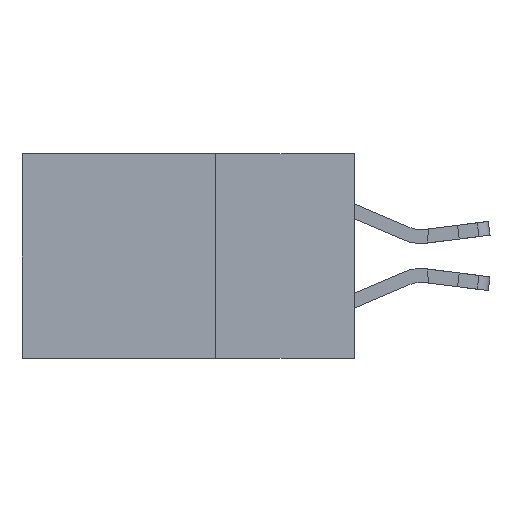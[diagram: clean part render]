
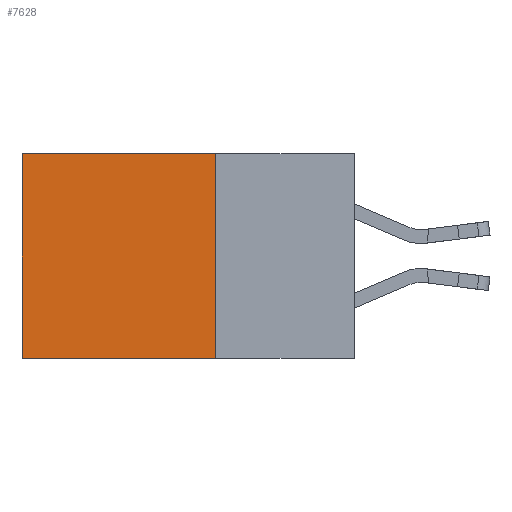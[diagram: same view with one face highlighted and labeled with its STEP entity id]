
A CAD part, left-side view. The second image highlights one B-rep face of the part: STEP entity #7628.
In plain terms, the highlighted planar face has unit normal (-1, 0, 0).
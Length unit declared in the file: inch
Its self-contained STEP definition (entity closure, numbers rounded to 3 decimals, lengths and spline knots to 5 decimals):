
#179 = ORIENTED_EDGE ( 'NONE', *, *, #23772, .T. ) ;
#721 = VECTOR ( 'NONE', #7195, 39.37008 ) ;
#1324 = LINE ( 'NONE', #23699, #721 ) ;
#1481 = DIRECTION ( 'NONE',  ( 0., 0., -1. ) ) ;
#2876 = VERTEX_POINT ( 'NONE', #16165 ) ;
#3820 = CARTESIAN_POINT ( 'NONE',  ( 0.2615, 0.25, -0.37 ) ) ;
#3831 = LINE ( 'NONE', #6799, #17981 ) ;
#3905 = DIRECTION ( 'NONE',  ( 0., 1., 0. ) ) ;
#5344 = EDGE_CURVE ( 'NONE', #5676, #2876, #20279, .T. ) ;
#5606 = VECTOR ( 'NONE', #3905, 39.37008 ) ;
#5676 = VERTEX_POINT ( 'NONE', #17682 ) ;
#6683 = CARTESIAN_POINT ( 'NONE',  ( 0.2615, 0.25, 0. ) ) ;
#6799 = CARTESIAN_POINT ( 'NONE',  ( 0.2615, 0.6, -0.37 ) ) ;
#7195 = DIRECTION ( 'NONE',  ( 0., 0., -1. ) ) ;
#7628 = ADVANCED_FACE ( 'NONE', ( #11336 ), #19925, .F. ) ;
#8099 = EDGE_LOOP ( 'NONE', ( #19903, #8812, #15203, #179 ) ) ;
#8812 = ORIENTED_EDGE ( 'NONE', *, *, #5344, .F. ) ;
#9086 = VERTEX_POINT ( 'NONE', #14521 ) ;
#11336 = FACE_OUTER_BOUND ( 'NONE', #8099, .T. ) ;
#12271 = VECTOR ( 'NONE', #17684, 39.37008 ) ;
#12656 = DIRECTION ( 'NONE',  ( 1., 0., 0. ) ) ;
#13134 = VERTEX_POINT ( 'NONE', #20858 ) ;
#14521 = CARTESIAN_POINT ( 'NONE',  ( 0.2615, 0.6, 0. ) ) ;
#15203 = ORIENTED_EDGE ( 'NONE', *, *, #22240, .F. ) ;
#16165 = CARTESIAN_POINT ( 'NONE',  ( 0.2615, 0.6, -0.37 ) ) ;
#17129 = LINE ( 'NONE', #6683, #12271 ) ;
#17682 = CARTESIAN_POINT ( 'NONE',  ( 0.2615, 0.25, -0.37 ) ) ;
#17684 = DIRECTION ( 'NONE',  ( 0., 1., 0. ) ) ;
#17981 = VECTOR ( 'NONE', #21470, 39.37008 ) ;
#19490 = EDGE_CURVE ( 'NONE', #9086, #2876, #3831, .T. ) ;
#19903 = ORIENTED_EDGE ( 'NONE', *, *, #19490, .T. ) ;
#19925 = PLANE ( 'NONE',  #20273 ) ;
#20273 = AXIS2_PLACEMENT_3D ( 'NONE', #21764, #12656, #1481 ) ;
#20279 = LINE ( 'NONE', #3820, #5606 ) ;
#20858 = CARTESIAN_POINT ( 'NONE',  ( 0.2615, 0.25, 0. ) ) ;
#21470 = DIRECTION ( 'NONE',  ( 0., 0., -1. ) ) ;
#21764 = CARTESIAN_POINT ( 'NONE',  ( 0.2615, 0.25, -0.37 ) ) ;
#22240 = EDGE_CURVE ( 'NONE', #13134, #5676, #1324, .T. ) ;
#23699 = CARTESIAN_POINT ( 'NONE',  ( 0.2615, 0.25, -0.37 ) ) ;
#23772 = EDGE_CURVE ( 'NONE', #13134, #9086, #17129, .T. ) ;
